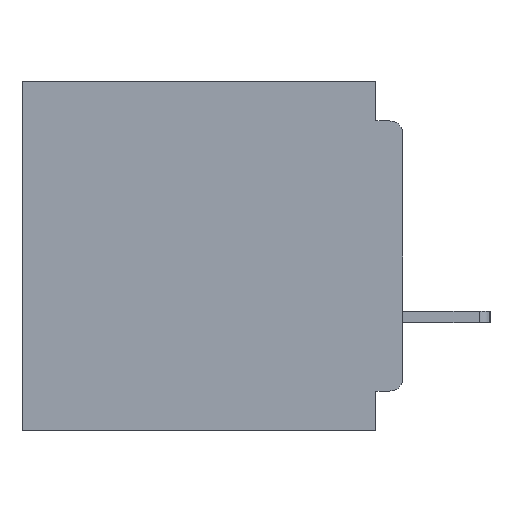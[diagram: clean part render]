
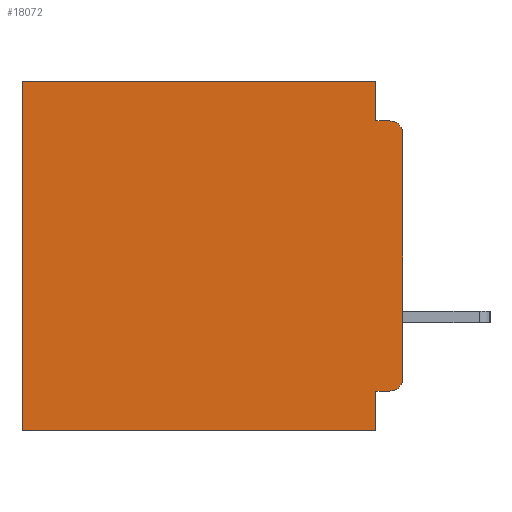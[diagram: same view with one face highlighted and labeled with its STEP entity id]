
A CAD part, left-side view. The second image highlights one B-rep face of the part: STEP entity #18072.
In plain terms, the highlighted planar face has unit normal (-1, 0, 0).
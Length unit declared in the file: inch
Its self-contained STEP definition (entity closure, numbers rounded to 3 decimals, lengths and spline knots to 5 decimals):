
#30 = DIRECTION ( 'NONE',  ( 0., 0., -1. ) ) ;
#64 = CARTESIAN_POINT ( 'NONE',  ( 0.3, 0., -0.4 ) ) ;
#123 = EDGE_CURVE ( 'NONE', #34455, #30213, #25128, .T. ) ;
#1359 = VERTEX_POINT ( 'NONE', #30221 ) ;
#1575 = LINE ( 'NONE', #64, #15852 ) ;
#1674 = CARTESIAN_POINT ( 'NONE',  ( 0.3, 0., 0. ) ) ;
#1763 = CARTESIAN_POINT ( 'NONE',  ( 0.3, 0.031, -0.045 ) ) ;
#4585 = ORIENTED_EDGE ( 'NONE', *, *, #9534, .T. ) ;
#4661 = EDGE_CURVE ( 'NONE', #34455, #14727, #28032, .T. ) ;
#4747 = DIRECTION ( 'NONE',  ( 1., 0., 0. ) ) ;
#5407 = CARTESIAN_POINT ( 'NONE',  ( 0.3, 0.437, -0.4 ) ) ;
#5450 = CARTESIAN_POINT ( 'NONE',  ( 0.3, 0.031, 0. ) ) ;
#5801 = CARTESIAN_POINT ( 'NONE',  ( 0.3, 0.031, -0.4 ) ) ;
#6460 = LINE ( 'NONE', #1674, #20646 ) ;
#7103 = CIRCLE ( 'NONE', #21759, 0.015 ) ;
#8098 = CARTESIAN_POINT ( 'NONE',  ( 0.3, 0.437, 0. ) ) ;
#8457 = DIRECTION ( 'NONE',  ( 0., 1., 0. ) ) ;
#8899 = CARTESIAN_POINT ( 'NONE',  ( 0.3, 0.015, -0.045 ) ) ;
#8983 = EDGE_CURVE ( 'NONE', #1359, #28438, #1575, .T. ) ;
#9534 = EDGE_CURVE ( 'NONE', #10782, #28438, #31233, .T. ) ;
#9675 = EDGE_CURVE ( 'NONE', #30213, #1359, #13606, .T. ) ;
#10013 = VERTEX_POINT ( 'NONE', #1763 ) ;
#10163 = DIRECTION ( 'NONE',  ( 0., -1., 0. ) ) ;
#10774 = DIRECTION ( 'NONE',  ( -1., 0., 0. ) ) ;
#10782 = VERTEX_POINT ( 'NONE', #8098 ) ;
#11927 = VECTOR ( 'NONE', #8457, 39.37008 ) ;
#12504 = DIRECTION ( 'NONE',  ( 0., 0., -1. ) ) ;
#12695 = VECTOR ( 'NONE', #30, 39.37008 ) ;
#13328 = DIRECTION ( 'NONE',  ( -1., 0., 0. ) ) ;
#13606 = LINE ( 'NONE', #5801, #12695 ) ;
#14259 = ORIENTED_EDGE ( 'NONE', *, *, #26048, .F. ) ;
#14342 = DIRECTION ( 'NONE',  ( 0., 1., 0. ) ) ;
#14421 = LINE ( 'NONE', #29429, #23674 ) ;
#14727 = VERTEX_POINT ( 'NONE', #27226 ) ;
#15142 = VECTOR ( 'NONE', #10163, 39.37008 ) ;
#15233 = ORIENTED_EDGE ( 'NONE', *, *, #4661, .T. ) ;
#15822 = AXIS2_PLACEMENT_3D ( 'NONE', #30205, #13328, #32999 ) ;
#15852 = VECTOR ( 'NONE', #14342, 39.37008 ) ;
#16296 = CARTESIAN_POINT ( 'NONE',  ( 0.3, 0., -0.355 ) ) ;
#16526 = VECTOR ( 'NONE', #12504, 39.37008 ) ;
#17263 = CARTESIAN_POINT ( 'NONE',  ( 0.3, 0.031, -0.355 ) ) ;
#17271 = EDGE_CURVE ( 'NONE', #30114, #10013, #14421, .T. ) ;
#17732 = ORIENTED_EDGE ( 'NONE', *, *, #26734, .F. ) ;
#18072 = ADVANCED_FACE ( 'NONE', ( #23601 ), #24459, .F. ) ;
#18076 = CARTESIAN_POINT ( 'NONE',  ( 0.3, 0.437, -0.4 ) ) ;
#19200 = AXIS2_PLACEMENT_3D ( 'NONE', #32948, #4747, #24581 ) ;
#19909 = EDGE_CURVE ( 'NONE', #34523, #29556, #7103, .T. ) ;
#20646 = VECTOR ( 'NONE', #21566, 39.37008 ) ;
#21414 = CARTESIAN_POINT ( 'NONE',  ( 0.3, 0., -0.045 ) ) ;
#21566 = DIRECTION ( 'NONE',  ( 0., 1., 0. ) ) ;
#21759 = AXIS2_PLACEMENT_3D ( 'NONE', #27661, #10774, #30535 ) ;
#23539 = LINE ( 'NONE', #21414, #15142 ) ;
#23601 = FACE_OUTER_BOUND ( 'NONE', #33280, .T. ) ;
#23674 = VECTOR ( 'NONE', #32260, 39.37008 ) ;
#23744 = VECTOR ( 'NONE', #25198, 39.37008 ) ;
#24459 = PLANE ( 'NONE',  #19200 ) ;
#24581 = DIRECTION ( 'NONE',  ( 0., 0., -1. ) ) ;
#24977 = ORIENTED_EDGE ( 'NONE', *, *, #8983, .F. ) ;
#25128 = LINE ( 'NONE', #16296, #11927 ) ;
#25198 = DIRECTION ( 'NONE',  ( 0., 0., -1. ) ) ;
#26048 = EDGE_CURVE ( 'NONE', #34523, #14727, #31506, .T. ) ;
#26734 = EDGE_CURVE ( 'NONE', #10013, #29556, #23539, .T. ) ;
#27226 = CARTESIAN_POINT ( 'NONE',  ( 0.3, 0., -0.34 ) ) ;
#27661 = CARTESIAN_POINT ( 'NONE',  ( 0.3, 0.015, -0.06 ) ) ;
#28032 = CIRCLE ( 'NONE', #15822, 0.015 ) ;
#28340 = ORIENTED_EDGE ( 'NONE', *, *, #123, .F. ) ;
#28438 = VERTEX_POINT ( 'NONE', #18076 ) ;
#28657 = CARTESIAN_POINT ( 'NONE',  ( 0.3, 0.015, -0.355 ) ) ;
#29429 = CARTESIAN_POINT ( 'NONE',  ( 0.3, 0.031, 0. ) ) ;
#29556 = VERTEX_POINT ( 'NONE', #8899 ) ;
#30114 = VERTEX_POINT ( 'NONE', #5450 ) ;
#30205 = CARTESIAN_POINT ( 'NONE',  ( 0.3, 0.015, -0.34 ) ) ;
#30213 = VERTEX_POINT ( 'NONE', #17263 ) ;
#30221 = CARTESIAN_POINT ( 'NONE',  ( 0.3, 0.031, -0.4 ) ) ;
#30535 = DIRECTION ( 'NONE',  ( 0., 0., -1. ) ) ;
#30540 = EDGE_CURVE ( 'NONE', #30114, #10782, #6460, .T. ) ;
#31233 = LINE ( 'NONE', #5407, #23744 ) ;
#31506 = LINE ( 'NONE', #35017, #16526 ) ;
#32260 = DIRECTION ( 'NONE',  ( 0., 0., -1. ) ) ;
#32948 = CARTESIAN_POINT ( 'NONE',  ( 0.3, 0., -0.4 ) ) ;
#32999 = DIRECTION ( 'NONE',  ( 0., 0., -1. ) ) ;
#33280 = EDGE_LOOP ( 'NONE', ( #14259, #34740, #17732, #33910, #34481, #4585, #24977, #35634, #28340, #15233 ) ) ;
#33910 = ORIENTED_EDGE ( 'NONE', *, *, #17271, .F. ) ;
#34455 = VERTEX_POINT ( 'NONE', #28657 ) ;
#34481 = ORIENTED_EDGE ( 'NONE', *, *, #30540, .T. ) ;
#34523 = VERTEX_POINT ( 'NONE', #34657 ) ;
#34657 = CARTESIAN_POINT ( 'NONE',  ( 0.3, 0., -0.06 ) ) ;
#34740 = ORIENTED_EDGE ( 'NONE', *, *, #19909, .T. ) ;
#35017 = CARTESIAN_POINT ( 'NONE',  ( 0.3, 0., -0.4 ) ) ;
#35634 = ORIENTED_EDGE ( 'NONE', *, *, #9675, .F. ) ;
